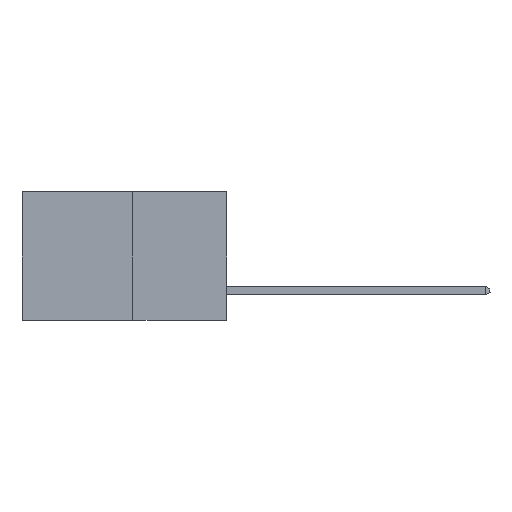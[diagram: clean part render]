
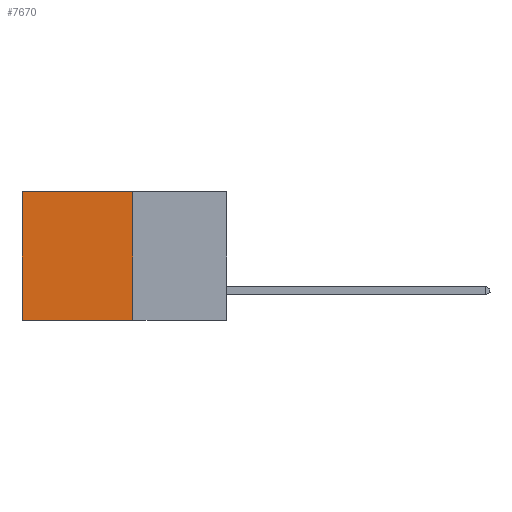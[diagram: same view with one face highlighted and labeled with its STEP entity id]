
A CAD part, left-side view. The second image highlights one B-rep face of the part: STEP entity #7670.
In plain terms, the highlighted planar face has unit normal (-1, 0, 0).
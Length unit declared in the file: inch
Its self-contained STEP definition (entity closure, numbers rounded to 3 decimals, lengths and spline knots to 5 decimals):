
#985 = EDGE_CURVE ( 'NONE', #7111, #9093, #13705, .T. ) ;
#1107 = CARTESIAN_POINT ( 'NONE',  ( 0.277, 0.27, 0. ) ) ;
#2694 = EDGE_LOOP ( 'NONE', ( #9277, #12037, #16515, #13526 ) ) ;
#3983 = EDGE_CURVE ( 'NONE', #16037, #7111, #15155, .T. ) ;
#4522 = VECTOR ( 'NONE', #5180, 39.37008 ) ;
#4677 = DIRECTION ( 'NONE',  ( 0., 0., -1. ) ) ;
#4683 = DIRECTION ( 'NONE',  ( 1., 0., 0. ) ) ;
#4749 = PLANE ( 'NONE',  #10160 ) ;
#4751 = VECTOR ( 'NONE', #5244, 39.37008 ) ;
#4924 = CARTESIAN_POINT ( 'NONE',  ( 0.277, 0.27, -0.37 ) ) ;
#5172 = DIRECTION ( 'NONE',  ( 0., 1., 0. ) ) ;
#5180 = DIRECTION ( 'NONE',  ( 0., 0., -1. ) ) ;
#5244 = DIRECTION ( 'NONE',  ( 0., 0., -1. ) ) ;
#5517 = CARTESIAN_POINT ( 'NONE',  ( 0.277, 0.27, -0.37 ) ) ;
#6742 = VECTOR ( 'NONE', #5172, 39.37008 ) ;
#7111 = VERTEX_POINT ( 'NONE', #11134 ) ;
#7610 = CARTESIAN_POINT ( 'NONE',  ( 0.277, 0.27, 0. ) ) ;
#7670 = ADVANCED_FACE ( 'NONE', ( #10285 ), #4749, .F. ) ;
#7793 = CARTESIAN_POINT ( 'NONE',  ( 0.277, 0.59, -0.37 ) ) ;
#8075 = LINE ( 'NONE', #7793, #4522 ) ;
#9093 = VERTEX_POINT ( 'NONE', #16084 ) ;
#9277 = ORIENTED_EDGE ( 'NONE', *, *, #16623, .T. ) ;
#10160 = AXIS2_PLACEMENT_3D ( 'NONE', #4924, #4683, #4677 ) ;
#10285 = FACE_OUTER_BOUND ( 'NONE', #2694, .T. ) ;
#11134 = CARTESIAN_POINT ( 'NONE',  ( 0.277, 0.27, -0.37 ) ) ;
#12037 = ORIENTED_EDGE ( 'NONE', *, *, #985, .F. ) ;
#12363 = VECTOR ( 'NONE', #16600, 39.37008 ) ;
#13526 = ORIENTED_EDGE ( 'NONE', *, *, #16525, .T. ) ;
#13705 = LINE ( 'NONE', #16820, #6742 ) ;
#13804 = CARTESIAN_POINT ( 'NONE',  ( 0.277, 0.59, 0. ) ) ;
#15155 = LINE ( 'NONE', #5517, #4751 ) ;
#15340 = LINE ( 'NONE', #7610, #12363 ) ;
#15755 = VERTEX_POINT ( 'NONE', #13804 ) ;
#16037 = VERTEX_POINT ( 'NONE', #1107 ) ;
#16084 = CARTESIAN_POINT ( 'NONE',  ( 0.277, 0.59, -0.37 ) ) ;
#16515 = ORIENTED_EDGE ( 'NONE', *, *, #3983, .F. ) ;
#16525 = EDGE_CURVE ( 'NONE', #16037, #15755, #15340, .T. ) ;
#16600 = DIRECTION ( 'NONE',  ( 0., 1., 0. ) ) ;
#16623 = EDGE_CURVE ( 'NONE', #15755, #9093, #8075, .T. ) ;
#16820 = CARTESIAN_POINT ( 'NONE',  ( 0.277, 0.27, -0.37 ) ) ;
